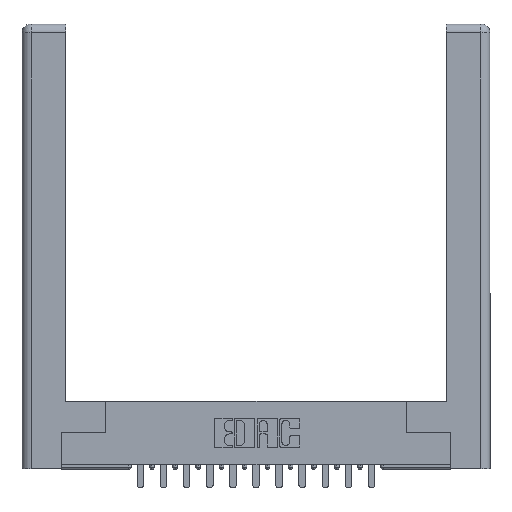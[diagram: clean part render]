
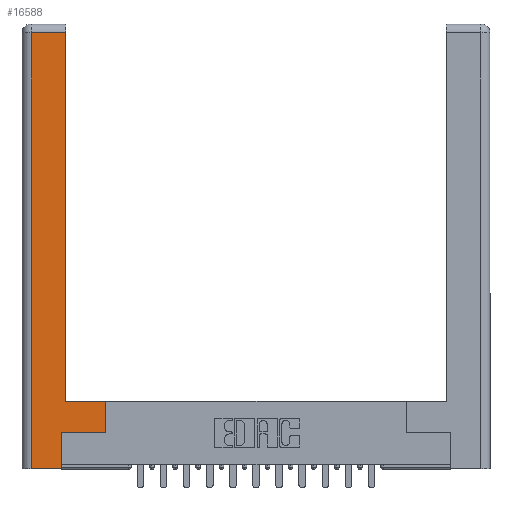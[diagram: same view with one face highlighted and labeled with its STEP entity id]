
A CAD part, top view. The second image highlights one B-rep face of the part: STEP entity #16588.
In plain terms, the highlighted planar face has unit normal (0, 0, 1).
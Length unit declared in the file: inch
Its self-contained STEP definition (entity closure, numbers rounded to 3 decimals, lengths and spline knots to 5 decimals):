
#51 = EDGE_CURVE ( 'NONE', #5090, #1289, #4342, .T. ) ;
#196 = ORIENTED_EDGE ( 'NONE', *, *, #1659, .T. ) ;
#269 = CARTESIAN_POINT ( 'NONE',  ( 0.565, 0.245, 0. ) ) ;
#340 = VERTEX_POINT ( 'NONE', #11186 ) ;
#539 = VERTEX_POINT ( 'NONE', #269 ) ;
#590 = VECTOR ( 'NONE', #15142, 39.37008 ) ;
#812 = DIRECTION ( 'NONE',  ( -1., 0., 0. ) ) ;
#1289 = VERTEX_POINT ( 'NONE', #10882 ) ;
#1382 = CARTESIAN_POINT ( 'NONE',  ( 0.0615, 2.94, 0. ) ) ;
#1437 = EDGE_CURVE ( 'NONE', #6108, #8386, #7395, .T. ) ;
#1588 = ORIENTED_EDGE ( 'NONE', *, *, #11432, .T. ) ;
#1659 = EDGE_CURVE ( 'NONE', #9619, #539, #16835, .T. ) ;
#1668 = LINE ( 'NONE', #7944, #6941 ) ;
#2184 = CARTESIAN_POINT ( 'NONE',  ( 0.295, 0.45, 0. ) ) ;
#2274 = CARTESIAN_POINT ( 'NONE',  ( 0.565, 0.245, 0. ) ) ;
#2374 = AXIS2_PLACEMENT_3D ( 'NONE', #7172, #7405, #3040 ) ;
#2606 = VERTEX_POINT ( 'NONE', #3167 ) ;
#2891 = LINE ( 'NONE', #15678, #8603 ) ;
#3040 = DIRECTION ( 'NONE',  ( -1., 0., 0. ) ) ;
#3167 = CARTESIAN_POINT ( 'NONE',  ( 0.265, 0., 0. ) ) ;
#3195 = EDGE_LOOP ( 'NONE', ( #17167, #10768, #9140, #14456, #1588, #196, #8530, #3635 ) ) ;
#3396 = CARTESIAN_POINT ( 'NONE',  ( 0.295, 2.94, 0. ) ) ;
#3561 = DIRECTION ( 'NONE',  ( 1., 0., 0. ) ) ;
#3635 = ORIENTED_EDGE ( 'NONE', *, *, #7648, .T. ) ;
#4342 = LINE ( 'NONE', #8311, #10727 ) ;
#5090 = VERTEX_POINT ( 'NONE', #1382 ) ;
#5411 = CARTESIAN_POINT ( 'NONE',  ( 0.565, 0.45, 0. ) ) ;
#5729 = DIRECTION ( 'NONE',  ( 0., 1., 0. ) ) ;
#6018 = FACE_OUTER_BOUND ( 'NONE', #3195, .T. ) ;
#6108 = VERTEX_POINT ( 'NONE', #12743 ) ;
#6941 = VECTOR ( 'NONE', #812, 39.37008 ) ;
#7172 = CARTESIAN_POINT ( 'NONE',  ( 0., 0., 0. ) ) ;
#7340 = EDGE_CURVE ( 'NONE', #539, #340, #15993, .T. ) ;
#7395 = LINE ( 'NONE', #10142, #18172 ) ;
#7405 = DIRECTION ( 'NONE',  ( 0., 0., -1. ) ) ;
#7648 = EDGE_CURVE ( 'NONE', #340, #6108, #17308, .T. ) ;
#7944 = CARTESIAN_POINT ( 'NONE',  ( 0.0615, 2.94, 0. ) ) ;
#8311 = CARTESIAN_POINT ( 'NONE',  ( 0.0615, 0., 0. ) ) ;
#8386 = VERTEX_POINT ( 'NONE', #3396 ) ;
#8530 = ORIENTED_EDGE ( 'NONE', *, *, #7340, .T. ) ;
#8603 = VECTOR ( 'NONE', #10058, 39.37008 ) ;
#9140 = ORIENTED_EDGE ( 'NONE', *, *, #51, .T. ) ;
#9619 = VERTEX_POINT ( 'NONE', #12176 ) ;
#10040 = PLANE ( 'NONE',  #2374 ) ;
#10058 = DIRECTION ( 'NONE',  ( 1., 0., 0. ) ) ;
#10142 = CARTESIAN_POINT ( 'NONE',  ( 0.295, 3., 0. ) ) ;
#10246 = VECTOR ( 'NONE', #13148, 39.37008 ) ;
#10727 = VECTOR ( 'NONE', #13866, 39.37008 ) ;
#10768 = ORIENTED_EDGE ( 'NONE', *, *, #15248, .T. ) ;
#10882 = CARTESIAN_POINT ( 'NONE',  ( 0.0615, 0., 0. ) ) ;
#11186 = CARTESIAN_POINT ( 'NONE',  ( 0.565, 0.45, 0. ) ) ;
#11432 = EDGE_CURVE ( 'NONE', #2606, #9619, #13998, .T. ) ;
#12014 = VECTOR ( 'NONE', #14678, 39.37008 ) ;
#12176 = CARTESIAN_POINT ( 'NONE',  ( 0.265, 0.245, 0. ) ) ;
#12743 = CARTESIAN_POINT ( 'NONE',  ( 0.295, 0.45, 0. ) ) ;
#13092 = VECTOR ( 'NONE', #3561, 39.37008 ) ;
#13148 = DIRECTION ( 'NONE',  ( 0., 1., 0. ) ) ;
#13866 = DIRECTION ( 'NONE',  ( 0., -1., 0. ) ) ;
#13998 = LINE ( 'NONE', #16116, #10246 ) ;
#14430 = EDGE_CURVE ( 'NONE', #1289, #2606, #2891, .T. ) ;
#14456 = ORIENTED_EDGE ( 'NONE', *, *, #14430, .T. ) ;
#14678 = DIRECTION ( 'NONE',  ( -1., 0., 0. ) ) ;
#15142 = DIRECTION ( 'NONE',  ( 0., 1., 0. ) ) ;
#15248 = EDGE_CURVE ( 'NONE', #8386, #5090, #1668, .T. ) ;
#15678 = CARTESIAN_POINT ( 'NONE',  ( 0.265, 0., 0. ) ) ;
#15993 = LINE ( 'NONE', #5411, #590 ) ;
#16116 = CARTESIAN_POINT ( 'NONE',  ( 0.265, 0.245, 0. ) ) ;
#16588 = ADVANCED_FACE ( 'NONE', ( #6018 ), #10040, .F. ) ;
#16835 = LINE ( 'NONE', #2274, #13092 ) ;
#17167 = ORIENTED_EDGE ( 'NONE', *, *, #1437, .T. ) ;
#17308 = LINE ( 'NONE', #2184, #12014 ) ;
#18172 = VECTOR ( 'NONE', #5729, 39.37008 ) ;
